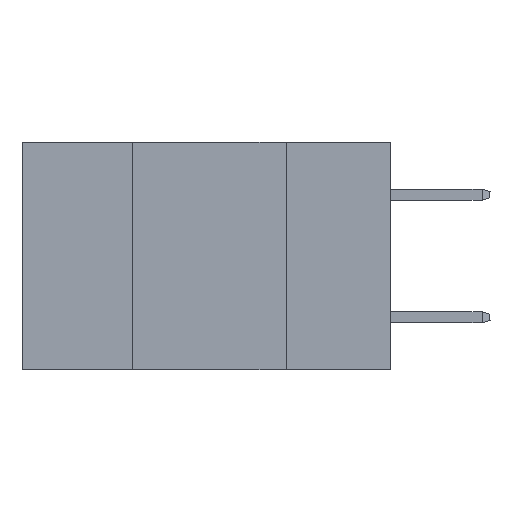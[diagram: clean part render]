
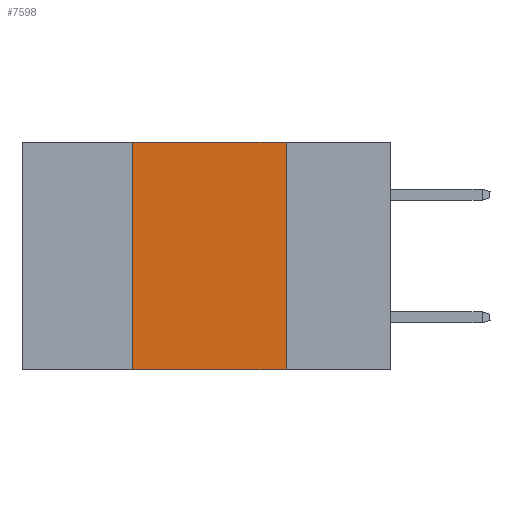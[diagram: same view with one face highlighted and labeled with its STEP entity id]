
A CAD part, left-side view. The second image highlights one B-rep face of the part: STEP entity #7598.
In plain terms, the highlighted planar face has unit normal (-1, 0, 0).
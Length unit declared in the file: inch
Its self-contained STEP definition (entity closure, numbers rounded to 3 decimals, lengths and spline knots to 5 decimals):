
#463 = PLANE ( 'NONE',  #15642 ) ;
#665 = CARTESIAN_POINT ( 'NONE',  ( 0., 0.17, -0.37 ) ) ;
#713 = CARTESIAN_POINT ( 'NONE',  ( 0., 0.6, 0. ) ) ;
#720 = DIRECTION ( 'NONE',  ( 0., 0., -1. ) ) ;
#1059 = LINE ( 'NONE', #11278, #1526 ) ;
#1526 = VECTOR ( 'NONE', #2408, 39.37008 ) ;
#2408 = DIRECTION ( 'NONE',  ( 0., 0., -1. ) ) ;
#3188 = CARTESIAN_POINT ( 'NONE',  ( 0., 0.6, 0. ) ) ;
#3683 = EDGE_CURVE ( 'NONE', #7436, #14408, #17777, .T. ) ;
#5095 = EDGE_CURVE ( 'NONE', #16968, #14408, #1059, .T. ) ;
#5293 = DIRECTION ( 'NONE',  ( 0., 0., 1. ) ) ;
#5833 = VECTOR ( 'NONE', #10359, 39.37008 ) ;
#6997 = CARTESIAN_POINT ( 'NONE',  ( 0., 0.6, -0.37 ) ) ;
#7131 = VECTOR ( 'NONE', #8160, 39.37008 ) ;
#7436 = VERTEX_POINT ( 'NONE', #18041 ) ;
#7598 = ADVANCED_FACE ( 'NONE', ( #8193 ), #463, .F. ) ;
#7977 = DIRECTION ( 'NONE',  ( 1., 0., 0. ) ) ;
#8160 = DIRECTION ( 'NONE',  ( 0., -1., 0. ) ) ;
#8193 = FACE_OUTER_BOUND ( 'NONE', #13690, .T. ) ;
#9408 = ORIENTED_EDGE ( 'NONE', *, *, #5095, .F. ) ;
#10359 = DIRECTION ( 'NONE',  ( 0., -1., 0. ) ) ;
#11045 = LINE ( 'NONE', #18693, #18841 ) ;
#11278 = CARTESIAN_POINT ( 'NONE',  ( 0., 0.17, 0. ) ) ;
#11426 = ORIENTED_EDGE ( 'NONE', *, *, #12621, .F. ) ;
#11959 = CARTESIAN_POINT ( 'NONE',  ( 0., 0.42, 0. ) ) ;
#12621 = EDGE_CURVE ( 'NONE', #18619, #16968, #17913, .T. ) ;
#13690 = EDGE_LOOP ( 'NONE', ( #9408, #11426, #16068, #18342 ) ) ;
#14408 = VERTEX_POINT ( 'NONE', #665 ) ;
#15642 = AXIS2_PLACEMENT_3D ( 'NONE', #3188, #7977, #720 ) ;
#16068 = ORIENTED_EDGE ( 'NONE', *, *, #16432, .F. ) ;
#16207 = CARTESIAN_POINT ( 'NONE',  ( 0., 0.17, 0. ) ) ;
#16432 = EDGE_CURVE ( 'NONE', #7436, #18619, #11045, .T. ) ;
#16968 = VERTEX_POINT ( 'NONE', #16207 ) ;
#17777 = LINE ( 'NONE', #6997, #5833 ) ;
#17913 = LINE ( 'NONE', #713, #7131 ) ;
#18041 = CARTESIAN_POINT ( 'NONE',  ( 0., 0.42, -0.37 ) ) ;
#18342 = ORIENTED_EDGE ( 'NONE', *, *, #3683, .T. ) ;
#18619 = VERTEX_POINT ( 'NONE', #11959 ) ;
#18693 = CARTESIAN_POINT ( 'NONE',  ( 0., 0.42, 0. ) ) ;
#18841 = VECTOR ( 'NONE', #5293, 39.37008 ) ;
